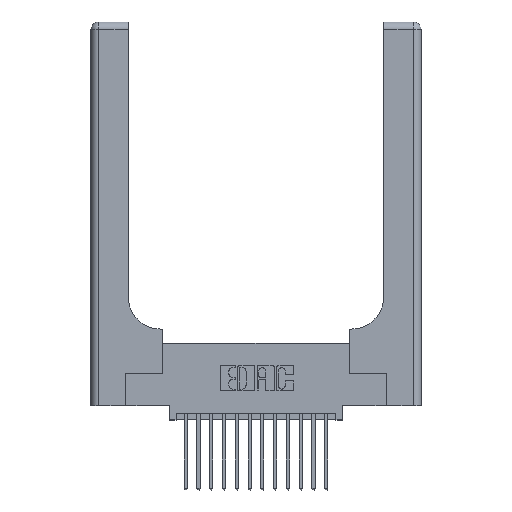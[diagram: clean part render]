
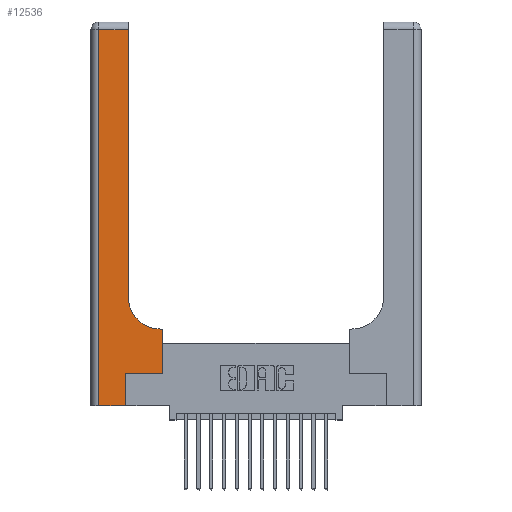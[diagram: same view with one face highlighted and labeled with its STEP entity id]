
A CAD part, top view. The second image highlights one B-rep face of the part: STEP entity #12536.
In plain terms, the highlighted planar face has unit normal (0, 0, 1).
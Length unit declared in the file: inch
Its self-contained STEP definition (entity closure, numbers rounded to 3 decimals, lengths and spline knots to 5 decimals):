
#199 = DIRECTION ( 'NONE',  ( -1., 0., 0. ) ) ;
#666 = CARTESIAN_POINT ( 'NONE',  ( 0.5415, 0.85, 0.37 ) ) ;
#1202 = EDGE_CURVE ( 'NONE', #15575, #8598, #3669, .T. ) ;
#1550 = EDGE_CURVE ( 'NONE', #8598, #8211, #5910, .T. ) ;
#1689 = ORIENTED_EDGE ( 'NONE', *, *, #10719, .T. ) ;
#1994 = LINE ( 'NONE', #14788, #16968 ) ;
#2144 = DIRECTION ( 'NONE',  ( 1., 0., 0. ) ) ;
#2723 = CARTESIAN_POINT ( 'NONE',  ( 0.269, 0.25, 0.37 ) ) ;
#2815 = ORIENTED_EDGE ( 'NONE', *, *, #6796, .T. ) ;
#2843 = CARTESIAN_POINT ( 'NONE',  ( 0.2915, 0.85, 0.37 ) ) ;
#3669 = LINE ( 'NONE', #10347, #14791 ) ;
#3829 = PLANE ( 'NONE',  #3993 ) ;
#3993 = AXIS2_PLACEMENT_3D ( 'NONE', #15430, #6726, #16865 ) ;
#4207 = CARTESIAN_POINT ( 'NONE',  ( 0.5585, 0.25, 0.37 ) ) ;
#4289 = LINE ( 'NONE', #11420, #16302 ) ;
#5122 = ORIENTED_EDGE ( 'NONE', *, *, #8286, .T. ) ;
#5862 = ORIENTED_EDGE ( 'NONE', *, *, #15573, .T. ) ;
#5910 = LINE ( 'NONE', #6579, #17465 ) ;
#6059 = DIRECTION ( 'NONE',  ( 0., 1., 0. ) ) ;
#6070 = FACE_OUTER_BOUND ( 'NONE', #14201, .T. ) ;
#6138 = VECTOR ( 'NONE', #199, 39.37008 ) ;
#6304 = EDGE_CURVE ( 'NONE', #8211, #10992, #13895, .T. ) ;
#6568 = LINE ( 'NONE', #16688, #7464 ) ;
#6579 = CARTESIAN_POINT ( 'NONE',  ( 0.2915, 0.6, 0.37 ) ) ;
#6605 = AXIS2_PLACEMENT_3D ( 'NONE', #666, #10867, #2144 ) ;
#6726 = DIRECTION ( 'NONE',  ( 0., 0., -1. ) ) ;
#6777 = DIRECTION ( 'NONE',  ( -1., 0., 0. ) ) ;
#6796 = EDGE_CURVE ( 'NONE', #18777, #6929, #13879, .T. ) ;
#6929 = VERTEX_POINT ( 'NONE', #12168 ) ;
#7103 = DIRECTION ( 'NONE',  ( 0., 1., 0. ) ) ;
#7464 = VECTOR ( 'NONE', #8024, 39.37008 ) ;
#7731 = ORIENTED_EDGE ( 'NONE', *, *, #1550, .T. ) ;
#8024 = DIRECTION ( 'NONE',  ( 0., -1., 0. ) ) ;
#8211 = VERTEX_POINT ( 'NONE', #16020 ) ;
#8286 = EDGE_CURVE ( 'NONE', #18313, #18468, #16097, .T. ) ;
#8598 = VERTEX_POINT ( 'NONE', #17210 ) ;
#8924 = CARTESIAN_POINT ( 'NONE',  ( 0., 2.94, 0.37 ) ) ;
#8998 = DIRECTION ( 'NONE',  ( 1., 0., 0. ) ) ;
#9520 = ORIENTED_EDGE ( 'NONE', *, *, #1202, .T. ) ;
#9967 = DIRECTION ( 'NONE',  ( 1., 0., 0. ) ) ;
#10113 = CARTESIAN_POINT ( 'NONE',  ( 0.269, 0., 0.37 ) ) ;
#10347 = CARTESIAN_POINT ( 'NONE',  ( 0.5585, 0.25, 0.37 ) ) ;
#10473 = DIRECTION ( 'NONE',  ( 0., 1., 0. ) ) ;
#10501 = VECTOR ( 'NONE', #9967, 39.37008 ) ;
#10719 = EDGE_CURVE ( 'NONE', #6929, #13723, #6568, .T. ) ;
#10867 = DIRECTION ( 'NONE',  ( 0., 0., -1. ) ) ;
#10992 = VERTEX_POINT ( 'NONE', #2843 ) ;
#11093 = ORIENTED_EDGE ( 'NONE', *, *, #17858, .T. ) ;
#11420 = CARTESIAN_POINT ( 'NONE',  ( 0.2915, 3., 0.37 ) ) ;
#12168 = CARTESIAN_POINT ( 'NONE',  ( 0.06, 2.94, 0.37 ) ) ;
#12263 = VECTOR ( 'NONE', #6059, 39.37008 ) ;
#12536 = ADVANCED_FACE ( 'NONE', ( #6070 ), #3829, .F. ) ;
#13400 = ORIENTED_EDGE ( 'NONE', *, *, #6304, .T. ) ;
#13723 = VERTEX_POINT ( 'NONE', #17000 ) ;
#13879 = LINE ( 'NONE', #8924, #6138 ) ;
#13895 = CIRCLE ( 'NONE', #6605, 0.25 ) ;
#14201 = EDGE_LOOP ( 'NONE', ( #17681, #2815, #1689, #11093, #5122, #5862, #9520, #7731, #13400 ) ) ;
#14788 = CARTESIAN_POINT ( 'NONE',  ( 0., 0., 0.37 ) ) ;
#14791 = VECTOR ( 'NONE', #10473, 39.37008 ) ;
#15430 = CARTESIAN_POINT ( 'NONE',  ( 0., 3., 0.37 ) ) ;
#15573 = EDGE_CURVE ( 'NONE', #18468, #15575, #18633, .T. ) ;
#15575 = VERTEX_POINT ( 'NONE', #4207 ) ;
#16020 = CARTESIAN_POINT ( 'NONE',  ( 0.5415, 0.6, 0.37 ) ) ;
#16097 = LINE ( 'NONE', #16147, #12263 ) ;
#16147 = CARTESIAN_POINT ( 'NONE',  ( 0.269, 0., 0.37 ) ) ;
#16195 = CARTESIAN_POINT ( 'NONE',  ( 0.269, 0.25, 0.37 ) ) ;
#16302 = VECTOR ( 'NONE', #7103, 39.37008 ) ;
#16688 = CARTESIAN_POINT ( 'NONE',  ( 0.06, 3., 0.37 ) ) ;
#16865 = DIRECTION ( 'NONE',  ( -1., 0., 0. ) ) ;
#16968 = VECTOR ( 'NONE', #8998, 39.37008 ) ;
#17000 = CARTESIAN_POINT ( 'NONE',  ( 0.06, 0., 0.37 ) ) ;
#17210 = CARTESIAN_POINT ( 'NONE',  ( 0.5585, 0.6, 0.37 ) ) ;
#17465 = VECTOR ( 'NONE', #6777, 39.37008 ) ;
#17681 = ORIENTED_EDGE ( 'NONE', *, *, #17693, .T. ) ;
#17693 = EDGE_CURVE ( 'NONE', #10992, #18777, #4289, .T. ) ;
#17858 = EDGE_CURVE ( 'NONE', #13723, #18313, #1994, .T. ) ;
#18313 = VERTEX_POINT ( 'NONE', #10113 ) ;
#18468 = VERTEX_POINT ( 'NONE', #16195 ) ;
#18556 = CARTESIAN_POINT ( 'NONE',  ( 0.2915, 2.94, 0.37 ) ) ;
#18633 = LINE ( 'NONE', #2723, #10501 ) ;
#18777 = VERTEX_POINT ( 'NONE', #18556 ) ;
